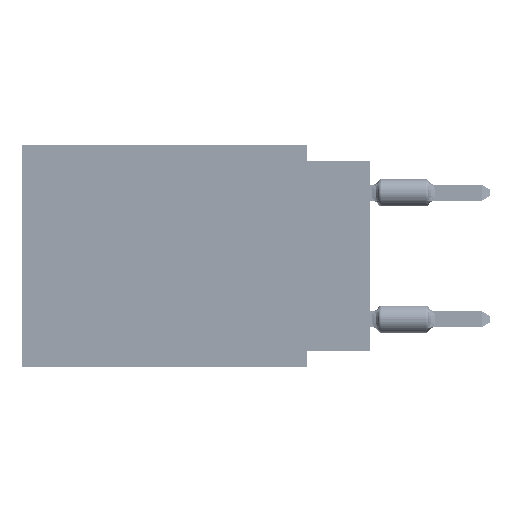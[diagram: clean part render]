
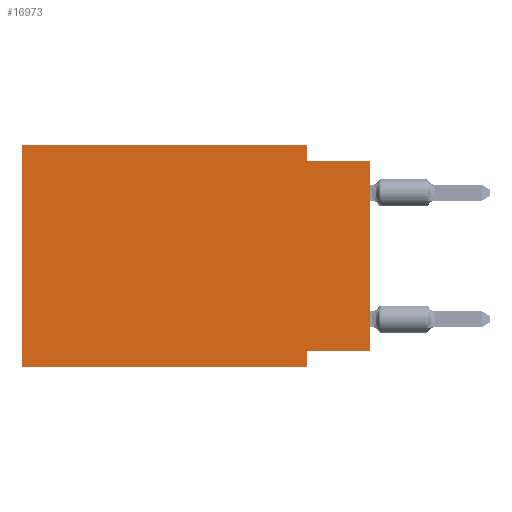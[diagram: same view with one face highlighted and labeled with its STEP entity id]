
A CAD part, left-side view. The second image highlights one B-rep face of the part: STEP entity #16973.
In plain terms, the highlighted planar face has unit normal (-1, 0, 0).
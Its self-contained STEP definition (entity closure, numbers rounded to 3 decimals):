
#1423 = VERTEX_POINT ( 'NONE', #5352 ) ;
#2183 = CARTESIAN_POINT ( 'NONE',  ( 0., 2.54, 0. ) ) ;
#2689 = CARTESIAN_POINT ( 'NONE',  ( 0., 0., -0.635 ) ) ;
#3119 = ORIENTED_EDGE ( 'NONE', *, *, #17767, .F. ) ;
#3512 = VECTOR ( 'NONE', #8315, 1000. ) ;
#5352 = CARTESIAN_POINT ( 'NONE',  ( 0., 2.54, 0. ) ) ;
#6498 = ORIENTED_EDGE ( 'NONE', *, *, #73925, .F. ) ;
#7242 = CARTESIAN_POINT ( 'NONE',  ( 0., 13.97, -8.89 ) ) ;
#7410 = CARTESIAN_POINT ( 'NONE',  ( 0., 2.54, -8.255 ) ) ;
#8315 = DIRECTION ( 'NONE',  ( 0., 1., 0. ) ) ;
#8900 = ORIENTED_EDGE ( 'NONE', *, *, #60694, .F. ) ;
#10108 = DIRECTION ( 'NONE',  ( 0., 0., -1. ) ) ;
#10419 = EDGE_CURVE ( 'NONE', #35653, #34774, #69170, .T. ) ;
#12189 = LINE ( 'NONE', #19180, #19348 ) ;
#12306 = ORIENTED_EDGE ( 'NONE', *, *, #32564, .F. ) ;
#15564 = DIRECTION ( 'NONE',  ( 1., 0., 0. ) ) ;
#16973 = ADVANCED_FACE ( 'NONE', ( #72982 ), #65964, .F. ) ;
#17767 = EDGE_CURVE ( 'NONE', #47535, #23196, #51751, .T. ) ;
#18143 = LINE ( 'NONE', #46621, #92076 ) ;
#18296 = DIRECTION ( 'NONE',  ( 0., 0., 1. ) ) ;
#19180 = CARTESIAN_POINT ( 'NONE',  ( 0., 13.97, 0. ) ) ;
#19348 = VECTOR ( 'NONE', #56057, 1000. ) ;
#22569 = ORIENTED_EDGE ( 'NONE', *, *, #10419, .F. ) ;
#23196 = VERTEX_POINT ( 'NONE', #90929 ) ;
#23456 = VECTOR ( 'NONE', #59191, 1000. ) ;
#24542 = DIRECTION ( 'NONE',  ( 0., 0., 1. ) ) ;
#27659 = VERTEX_POINT ( 'NONE', #82442 ) ;
#29121 = CARTESIAN_POINT ( 'NONE',  ( 0., 13.97, 0. ) ) ;
#30259 = CARTESIAN_POINT ( 'NONE',  ( 0., 0., -8.255 ) ) ;
#32347 = DIRECTION ( 'NONE',  ( 0., 0., -1. ) ) ;
#32564 = EDGE_CURVE ( 'NONE', #53788, #27659, #90705, .T. ) ;
#34774 = VERTEX_POINT ( 'NONE', #49104 ) ;
#34816 = DIRECTION ( 'NONE',  ( 0., -1., 0. ) ) ;
#35653 = VERTEX_POINT ( 'NONE', #62278 ) ;
#38577 = LINE ( 'NONE', #2183, #50829 ) ;
#41831 = LINE ( 'NONE', #7242, #80394 ) ;
#41970 = ORIENTED_EDGE ( 'NONE', *, *, #56779, .F. ) ;
#42999 = ORIENTED_EDGE ( 'NONE', *, *, #48728, .T. ) ;
#43985 = CARTESIAN_POINT ( 'NONE',  ( 0., 0., -8.255 ) ) ;
#46621 = CARTESIAN_POINT ( 'NONE',  ( 0., 0., 0. ) ) ;
#47535 = VERTEX_POINT ( 'NONE', #84356 ) ;
#48728 = EDGE_CURVE ( 'NONE', #35653, #27659, #41831, .T. ) ;
#49104 = CARTESIAN_POINT ( 'NONE',  ( 0., 13.97, 0. ) ) ;
#50829 = VECTOR ( 'NONE', #10108, 1000. ) ;
#51507 = DIRECTION ( 'NONE',  ( 0., 0., -1. ) ) ;
#51751 = LINE ( 'NONE', #2689, #23456 ) ;
#53788 = VERTEX_POINT ( 'NONE', #7410 ) ;
#56057 = DIRECTION ( 'NONE',  ( 0., -1., 0. ) ) ;
#56779 = EDGE_CURVE ( 'NONE', #34774, #1423, #12189, .T. ) ;
#57285 = VECTOR ( 'NONE', #32347, 1000. ) ;
#59191 = DIRECTION ( 'NONE',  ( 0., -1., 0. ) ) ;
#60694 = EDGE_CURVE ( 'NONE', #70465, #53788, #79754, .T. ) ;
#61188 = EDGE_LOOP ( 'NONE', ( #78615, #3119, #6498, #41970, #22569, #42999, #12306, #8900 ) ) ;
#61732 = CARTESIAN_POINT ( 'NONE',  ( 0., 2.54, -8.89 ) ) ;
#62278 = CARTESIAN_POINT ( 'NONE',  ( 0., 13.97, -8.89 ) ) ;
#65964 = PLANE ( 'NONE',  #88915 ) ;
#68277 = EDGE_CURVE ( 'NONE', #70465, #23196, #18143, .T. ) ;
#69170 = LINE ( 'NONE', #89274, #83244 ) ;
#70465 = VERTEX_POINT ( 'NONE', #43985 ) ;
#72982 = FACE_OUTER_BOUND ( 'NONE', #61188, .T. ) ;
#73925 = EDGE_CURVE ( 'NONE', #1423, #47535, #38577, .T. ) ;
#78615 = ORIENTED_EDGE ( 'NONE', *, *, #68277, .T. ) ;
#79754 = LINE ( 'NONE', #30259, #3512 ) ;
#80394 = VECTOR ( 'NONE', #34816, 1000. ) ;
#82442 = CARTESIAN_POINT ( 'NONE',  ( 0., 2.54, -8.89 ) ) ;
#83244 = VECTOR ( 'NONE', #18296, 1000. ) ;
#84356 = CARTESIAN_POINT ( 'NONE',  ( 0., 2.54, -0.635 ) ) ;
#88915 = AXIS2_PLACEMENT_3D ( 'NONE', #29121, #15564, #51507 ) ;
#89274 = CARTESIAN_POINT ( 'NONE',  ( 0., 13.97, 0. ) ) ;
#90705 = LINE ( 'NONE', #61732, #57285 ) ;
#90929 = CARTESIAN_POINT ( 'NONE',  ( 0., 0., -0.635 ) ) ;
#92076 = VECTOR ( 'NONE', #24542, 1000. ) ;
